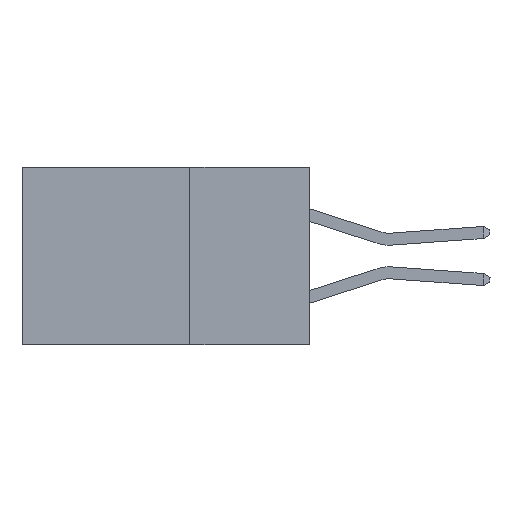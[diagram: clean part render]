
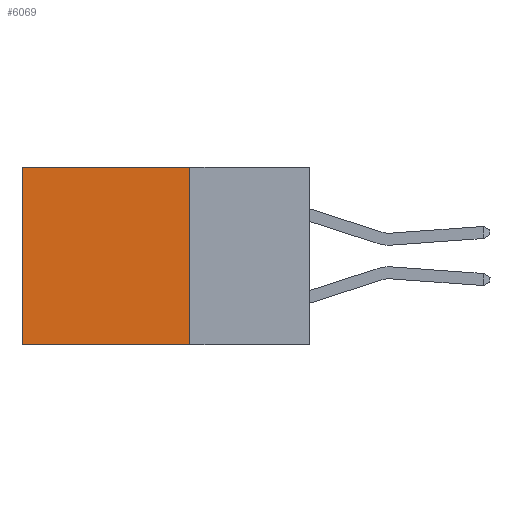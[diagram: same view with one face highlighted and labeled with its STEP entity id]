
A CAD part, left-side view. The second image highlights one B-rep face of the part: STEP entity #6069.
In plain terms, the highlighted planar face has unit normal (-1, 0, 0).
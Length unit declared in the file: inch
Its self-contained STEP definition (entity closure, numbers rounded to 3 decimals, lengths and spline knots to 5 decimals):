
#1 = LINE ( 'NONE', #15288, #15152 ) ;
#527 = CARTESIAN_POINT ( 'NONE',  ( 0.298, 0.25, 0. ) ) ;
#1072 = LINE ( 'NONE', #12159, #12313 ) ;
#1558 = VERTEX_POINT ( 'NONE', #3096 ) ;
#1845 = ORIENTED_EDGE ( 'NONE', *, *, #16612, .F. ) ;
#2938 = CARTESIAN_POINT ( 'NONE',  ( 0.298, 0.25, 0. ) ) ;
#3096 = CARTESIAN_POINT ( 'NONE',  ( 0.298, 0.25, -0.37 ) ) ;
#3098 = FACE_OUTER_BOUND ( 'NONE', #13412, .T. ) ;
#4094 = EDGE_CURVE ( 'NONE', #7813, #13351, #1072, .T. ) ;
#4756 = DIRECTION ( 'NONE',  ( 0., 0., -1. ) ) ;
#6069 = ADVANCED_FACE ( 'NONE', ( #3098 ), #9305, .F. ) ;
#7195 = VECTOR ( 'NONE', #14639, 39.37008 ) ;
#7743 = AXIS2_PLACEMENT_3D ( 'NONE', #527, #15434, #12566 ) ;
#7813 = VERTEX_POINT ( 'NONE', #16701 ) ;
#8761 = LINE ( 'NONE', #2938, #7195 ) ;
#9305 = PLANE ( 'NONE',  #7743 ) ;
#10206 = CARTESIAN_POINT ( 'NONE',  ( 0.298, 0.25, 0. ) ) ;
#10471 = DIRECTION ( 'NONE',  ( 0., 0., -1. ) ) ;
#11721 = EDGE_CURVE ( 'NONE', #18376, #7813, #8761, .T. ) ;
#12159 = CARTESIAN_POINT ( 'NONE',  ( 0.298, 0.6, 0. ) ) ;
#12313 = VECTOR ( 'NONE', #4756, 39.37008 ) ;
#12566 = DIRECTION ( 'NONE',  ( 0., 0., -1. ) ) ;
#13217 = ORIENTED_EDGE ( 'NONE', *, *, #4094, .T. ) ;
#13351 = VERTEX_POINT ( 'NONE', #13964 ) ;
#13412 = EDGE_LOOP ( 'NONE', ( #13217, #1845, #18379, #16153 ) ) ;
#13438 = CARTESIAN_POINT ( 'NONE',  ( 0.298, 0.25, 0. ) ) ;
#13836 = DIRECTION ( 'NONE',  ( 0., 1., 0. ) ) ;
#13854 = LINE ( 'NONE', #10206, #18660 ) ;
#13964 = CARTESIAN_POINT ( 'NONE',  ( 0.298, 0.6, -0.37 ) ) ;
#14639 = DIRECTION ( 'NONE',  ( 0., 1., 0. ) ) ;
#14875 = EDGE_CURVE ( 'NONE', #18376, #1558, #13854, .T. ) ;
#15152 = VECTOR ( 'NONE', #13836, 39.37008 ) ;
#15288 = CARTESIAN_POINT ( 'NONE',  ( 0.298, 0.25, -0.37 ) ) ;
#15434 = DIRECTION ( 'NONE',  ( 1., 0., 0. ) ) ;
#16153 = ORIENTED_EDGE ( 'NONE', *, *, #11721, .T. ) ;
#16612 = EDGE_CURVE ( 'NONE', #1558, #13351, #1, .T. ) ;
#16701 = CARTESIAN_POINT ( 'NONE',  ( 0.298, 0.6, 0. ) ) ;
#18376 = VERTEX_POINT ( 'NONE', #13438 ) ;
#18379 = ORIENTED_EDGE ( 'NONE', *, *, #14875, .F. ) ;
#18660 = VECTOR ( 'NONE', #10471, 39.37008 ) ;
